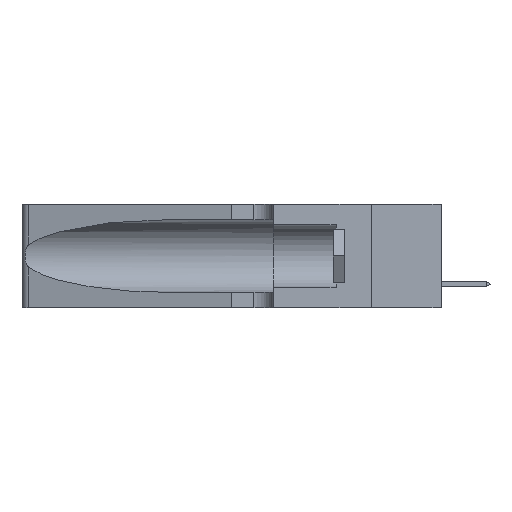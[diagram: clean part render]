
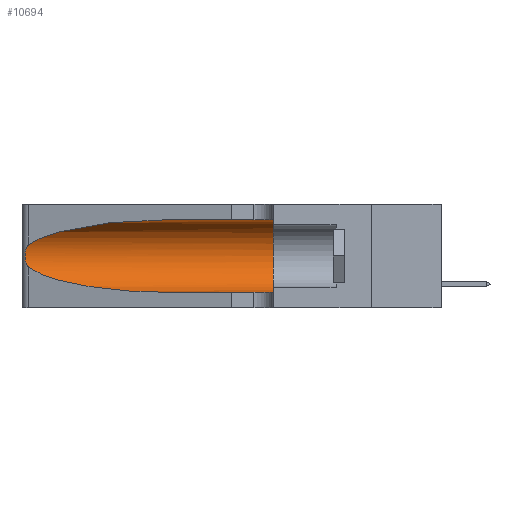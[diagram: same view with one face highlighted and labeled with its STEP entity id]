
A CAD part, left-side view. The second image highlights one B-rep face of the part: STEP entity #10694.
In plain terms, the highlighted cylindrical face has radius 3.308 mm (diameter 6.617 mm), a partial arc.
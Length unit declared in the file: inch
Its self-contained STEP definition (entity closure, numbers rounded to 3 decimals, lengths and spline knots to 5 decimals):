
#231 = CARTESIAN_POINT ( 'NONE',  ( 0.26075, 1.23896, 0.19203 ) ) ;
#297 = VECTOR ( 'NONE', #4201, 39.37008 ) ;
#555 =( BOUNDED_CURVE ( )  B_SPLINE_CURVE ( 3, ( #10517, #14295, #11673, #3701 ),
 .UNSPECIFIED., .F., .F. ) 
 B_SPLINE_CURVE_WITH_KNOTS ( ( 4, 4 ),
 ( 1.5708, 2.84003 ),
 .UNSPECIFIED. ) 
 CURVE ( )  GEOMETRIC_REPRESENTATION_ITEM ( )  RATIONAL_B_SPLINE_CURVE ( ( 1., 0.87, 0.87, 1. ) ) 
 REPRESENTATION_ITEM ( '' )  );
#732 = VERTEX_POINT ( 'NONE', #7451 ) ;
#1054 = DIRECTION ( 'NONE',  ( 0., 0., -1. ) ) ;
#1184 = CYLINDRICAL_SURFACE ( 'NONE', #8375, 0.13025 ) ;
#1342 = ORIENTED_EDGE ( 'NONE', *, *, #1855, .T. ) ;
#1347 = LINE ( 'NONE', #11937, #297 ) ;
#1353 = CARTESIAN_POINT ( 'NONE',  ( 0.25856, 1.23593, 0.16098 ) ) ;
#1364 = CARTESIAN_POINT ( 'NONE',  ( 0.2373, 1.15595, 0.08982 ) ) ;
#1579 = CARTESIAN_POINT ( 'NONE',  ( 0.25555, 1.22993, 0.14849 ) ) ;
#1590 = CARTESIAN_POINT ( 'NONE',  ( 0.18966, 0.96281, 0.05475 ) ) ;
#1855 = EDGE_CURVE ( 'NONE', #13699, #11194, #16017, .T. ) ;
#1934 = CARTESIAN_POINT ( 'NONE',  ( 0.25487, 1.22718, 0.22369 ) ) ;
#2223 = EDGE_CURVE ( 'NONE', #11194, #732, #3459, .T. ) ;
#2409 = EDGE_CURVE ( 'NONE', #14522, #10592, #1347, .T. ) ;
#2533 = CARTESIAN_POINT ( 'NONE',  ( 0.1305, 1.61858, 0.185 ) ) ;
#2875 = CARTESIAN_POINT ( 'NONE',  ( 0.25787, 1.23484, 0.2124 ) ) ;
#2942 = CARTESIAN_POINT ( 'NONE',  ( 0.26075, 1.23896, 0.178 ) ) ;
#2945 = EDGE_CURVE ( 'NONE', #14522, #17067, #555, .T. ) ;
#3126 = ORIENTED_EDGE ( 'NONE', *, *, #9910, .F. ) ;
#3459 = LINE ( 'NONE', #7298, #13427 ) ;
#3552 = CARTESIAN_POINT ( 'NONE',  ( 0.1305, 0.35, 0.185 ) ) ;
#3701 = CARTESIAN_POINT ( 'NONE',  ( 0.25487, 1.22718, 0.22369 ) ) ;
#4048 = CARTESIAN_POINT ( 'NONE',  ( 0.25555, 1.22994, 0.2215 ) ) ;
#4201 = DIRECTION ( 'NONE',  ( 0., -1., 0. ) ) ;
#4226 = CARTESIAN_POINT ( 'NONE',  ( 0.25854, 1.2359, 0.20912 ) ) ;
#5025 = CARTESIAN_POINT ( 'NONE',  ( 0.1305, 0.72297, 0.05475 ) ) ;
#6973 = CARTESIAN_POINT ( 'NONE',  ( 0.25639, 1.23184, 0.21858 ) ) ;
#7061 = FACE_OUTER_BOUND ( 'NONE', #9570, .T. ) ;
#7298 = CARTESIAN_POINT ( 'NONE',  ( 0.1305, 1.61858, 0.05475 ) ) ;
#7451 = CARTESIAN_POINT ( 'NONE',  ( 0.1305, 0.35, 0.05475 ) ) ;
#7556 = ORIENTED_EDGE ( 'NONE', *, *, #13754, .T. ) ;
#7922 = CIRCLE ( 'NONE', #9045, 0.13025 ) ;
#8375 = AXIS2_PLACEMENT_3D ( 'NONE', #2533, #13225, #1054 ) ;
#8480 = ORIENTED_EDGE ( 'NONE', *, *, #2223, .T. ) ;
#8652 = DIRECTION ( 'NONE',  ( 0., -1., 0. ) ) ;
#9045 = AXIS2_PLACEMENT_3D ( 'NONE', #3552, #11306, #12610 ) ;
#9570 = EDGE_LOOP ( 'NONE', ( #12876, #7556, #1342, #8480, #3126, #14240 ) ) ;
#9588 = CARTESIAN_POINT ( 'NONE',  ( 0.25639, 1.23186, 0.15144 ) ) ;
#9600 = CARTESIAN_POINT ( 'NONE',  ( 0.25487, 1.22718, 0.14631 ) ) ;
#9910 = EDGE_CURVE ( 'NONE', #10592, #732, #7922, .T. ) ;
#10294 = CARTESIAN_POINT ( 'NONE',  ( 0.1305, 0.35, 0.31525 ) ) ;
#10517 = CARTESIAN_POINT ( 'NONE',  ( 0.1305, 0.72297, 0.31525 ) ) ;
#10592 = VERTEX_POINT ( 'NONE', #10294 ) ;
#10694 = ADVANCED_FACE ( 'NONE', ( #7061 ), #1184, .F. ) ;
#10705 = CARTESIAN_POINT ( 'NONE',  ( 0.1305, 0.72297, 0.05475 ) ) ;
#10921 = CARTESIAN_POINT ( 'NONE',  ( 0.25487, 1.22718, 0.22369 ) ) ;
#11194 = VERTEX_POINT ( 'NONE', #5025 ) ;
#11306 = DIRECTION ( 'NONE',  ( 0., 1., 0. ) ) ;
#11673 = CARTESIAN_POINT ( 'NONE',  ( 0.2373, 1.15595, 0.28018 ) ) ;
#11937 = CARTESIAN_POINT ( 'NONE',  ( 0.1305, 1.61858, 0.31525 ) ) ;
#12509 = B_SPLINE_CURVE_WITH_KNOTS ( 'NONE', 3,
 ( #10921, #4048, #6973, #2875, #4226, #14816, #231, #2942, #14643, #1353, #13554, #9588, #1579, #16217 ),
 .UNSPECIFIED., .F., .F.,
 ( 4, 2, 2, 2, 2, 2, 4 ),
 ( 0., 0.00027, 0.00053, 0.00107, 0.0016, 0.00187, 0.00214 ),
 .UNSPECIFIED. ) ;
#12610 = DIRECTION ( 'NONE',  ( 0., 0., 1. ) ) ;
#12876 = ORIENTED_EDGE ( 'NONE', *, *, #2945, .T. ) ;
#13225 = DIRECTION ( 'NONE',  ( 0., -1., 0. ) ) ;
#13427 = VECTOR ( 'NONE', #8652, 39.37008 ) ;
#13554 = CARTESIAN_POINT ( 'NONE',  ( 0.25789, 1.23486, 0.15765 ) ) ;
#13699 = VERTEX_POINT ( 'NONE', #15866 ) ;
#13754 = EDGE_CURVE ( 'NONE', #17067, #13699, #12509, .T. ) ;
#14240 = ORIENTED_EDGE ( 'NONE', *, *, #2409, .F. ) ;
#14295 = CARTESIAN_POINT ( 'NONE',  ( 0.18966, 0.96281, 0.31525 ) ) ;
#14522 = VERTEX_POINT ( 'NONE', #15429 ) ;
#14643 = CARTESIAN_POINT ( 'NONE',  ( 0.26017, 1.23833, 0.17102 ) ) ;
#14816 = CARTESIAN_POINT ( 'NONE',  ( 0.26018, 1.23835, 0.19895 ) ) ;
#15429 = CARTESIAN_POINT ( 'NONE',  ( 0.1305, 0.72297, 0.31525 ) ) ;
#15866 = CARTESIAN_POINT ( 'NONE',  ( 0.25487, 1.22718, 0.14631 ) ) ;
#16017 =( BOUNDED_CURVE ( )  B_SPLINE_CURVE ( 3, ( #9600, #1364, #1590, #10705 ),
 .UNSPECIFIED., .F., .T. ) 
 B_SPLINE_CURVE_WITH_KNOTS ( ( 4, 4 ),
 ( 3.44316, 4.71239 ),
 .UNSPECIFIED. ) 
 CURVE ( )  GEOMETRIC_REPRESENTATION_ITEM ( )  RATIONAL_B_SPLINE_CURVE ( ( 1., 0.87, 0.87, 1. ) ) 
 REPRESENTATION_ITEM ( '' )  );
#16217 = CARTESIAN_POINT ( 'NONE',  ( 0.25487, 1.22718, 0.14631 ) ) ;
#17067 = VERTEX_POINT ( 'NONE', #1934 ) ;
